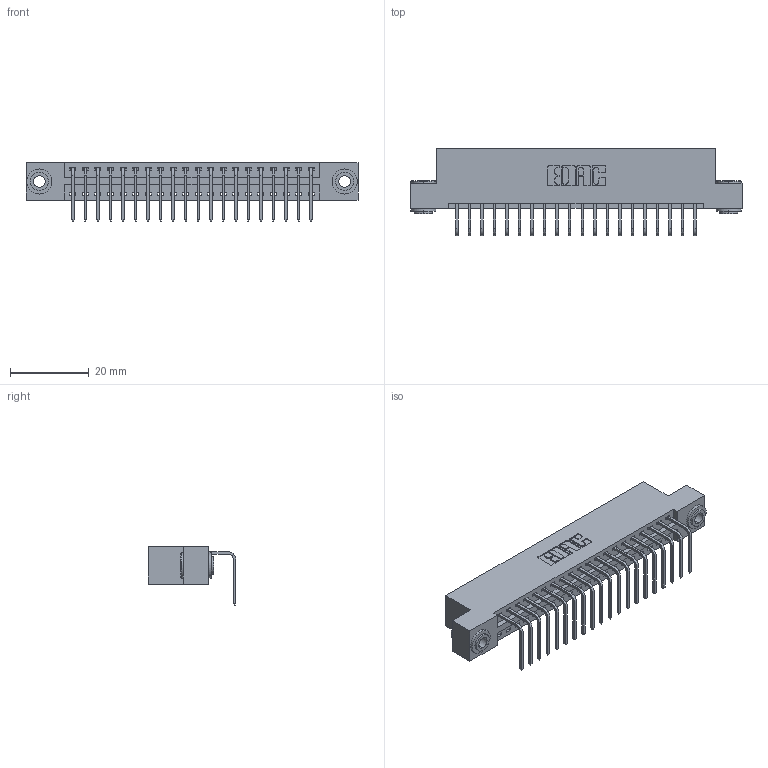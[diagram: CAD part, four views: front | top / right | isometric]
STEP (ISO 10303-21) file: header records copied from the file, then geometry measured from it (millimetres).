
FILE_DESCRIPTION (( 'STEP AP203' ), '1' );
FILE_NAME ('396-020-558-103.STEP', '2019-11-01T06:07:44', ( '' ), ( '' ), 'SwSTEP 2.0', 'SolidWorks 2016', '' );
FILE_SCHEMA (( 'CONFIG_CONTROL_DESIGN' ));
Length unit declared in the file: inch
Products named in the file (4): 345-250-002_345-250-002-102; 396-020-558-103; 346 Part_Flush Mounting Lugs - 0.156 Dia-TH; 345-292-001_558 Tail - 2
Assembly tree (23 placements, depth 2):
  396-020-558-103
    346 Part_Flush Mounting Lugs - 0.156 Dia-TH
    345-292-001_558 Tail - 2  x20
    345-250-002_345-250-002-102  x2
Bounding box: 84.07 x 22.16 x 14.73 mm (x, y, z)
Volume: 7982.2 mm3; surface area: 10356 mm2
Topology: 23 solids, 23 shells, 1360 faces, 4045 edges, 2666 vertices
Faces by surface type: plane 926, cylinder 426, cone 8
Entity records: 16108 total; most frequent: CARTESIAN_POINT 2747, ORIENTED_EDGE 2694, DIRECTION 2481, EDGE_CURVE 1347, VECTOR 1111, LINE 1111, VERTEX_POINT 894, AXIS2_PLACEMENT_3D 685
